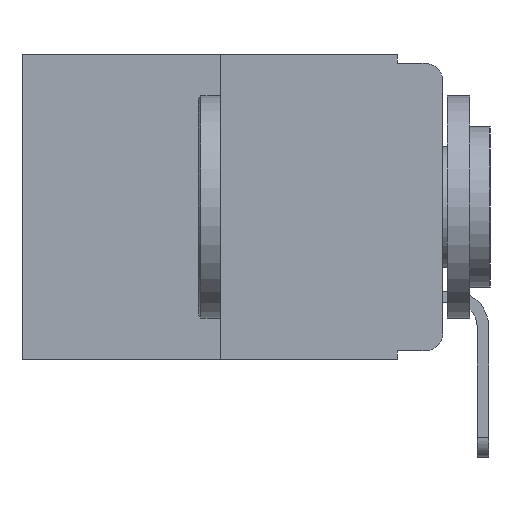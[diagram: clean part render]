
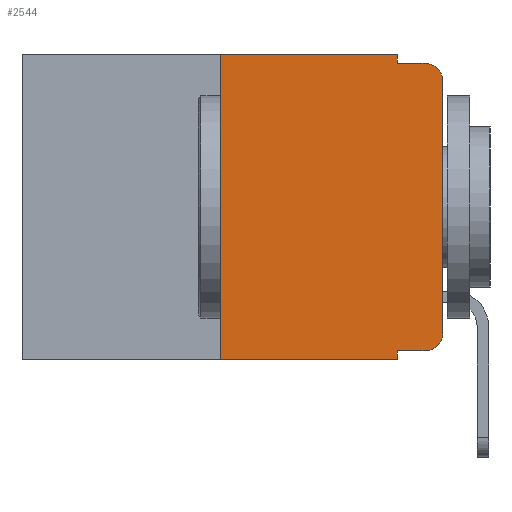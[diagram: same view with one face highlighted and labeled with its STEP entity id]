
A CAD part, left-side view. The second image highlights one B-rep face of the part: STEP entity #2544.
In plain terms, the highlighted planar face has unit normal (-1, 0, 0).
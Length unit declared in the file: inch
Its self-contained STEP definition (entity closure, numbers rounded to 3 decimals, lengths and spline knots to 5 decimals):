
#89 = VECTOR ( 'NONE', #8722, 39.37008 ) ;
#378 = AXIS2_PLACEMENT_3D ( 'NONE', #6134, #6126, #6123 ) ;
#442 = LINE ( 'NONE', #8966, #89 ) ;
#578 = VERTEX_POINT ( 'NONE', #7515 ) ;
#879 = ORIENTED_EDGE ( 'NONE', *, *, #8832, .T. ) ;
#962 = VERTEX_POINT ( 'NONE', #5371 ) ;
#1253 = ORIENTED_EDGE ( 'NONE', *, *, #8897, .T. ) ;
#1318 = CIRCLE ( 'NONE', #2718, 0.02 ) ;
#1372 = CARTESIAN_POINT ( 'NONE',  ( 0., 0.051, -0.333 ) ) ;
#1581 = CARTESIAN_POINT ( 'NONE',  ( 0., 0.25, -0.343 ) ) ;
#1769 = ORIENTED_EDGE ( 'NONE', *, *, #9022, .F. ) ;
#2022 = CARTESIAN_POINT ( 'NONE',  ( 0., 0., -0.313 ) ) ;
#2197 = ORIENTED_EDGE ( 'NONE', *, *, #9040, .F. ) ;
#2234 = ORIENTED_EDGE ( 'NONE', *, *, #4194, .F. ) ;
#2363 = CARTESIAN_POINT ( 'NONE',  ( 0., 0.051, -0.01 ) ) ;
#2544 = ADVANCED_FACE ( 'NONE', ( #10579 ), #7203, .F. ) ;
#2718 = AXIS2_PLACEMENT_3D ( 'NONE', #5008, #4945, #4886 ) ;
#2721 = CARTESIAN_POINT ( 'NONE',  ( 0., 0.051, -0.343 ) ) ;
#2747 = ORIENTED_EDGE ( 'NONE', *, *, #9093, .F. ) ;
#3010 = DIRECTION ( 'NONE',  ( 0., -1., 0. ) ) ;
#3046 = ORIENTED_EDGE ( 'NONE', *, *, #6772, .T. ) ;
#3079 = ORIENTED_EDGE ( 'NONE', *, *, #9110, .F. ) ;
#3125 = VERTEX_POINT ( 'NONE', #6711 ) ;
#3234 = EDGE_LOOP ( 'NONE', ( #879, #1253, #1769, #2197, #2234, #2747, #3046, #3079, #3517, #4168 ) ) ;
#3283 = LINE ( 'NONE', #8925, #7802 ) ;
#3517 = ORIENTED_EDGE ( 'NONE', *, *, #9247, .T. ) ;
#3841 = VECTOR ( 'NONE', #10121, 39.37008 ) ;
#3994 = CARTESIAN_POINT ( 'NONE',  ( 0., 0.051, 0. ) ) ;
#4105 = LINE ( 'NONE', #10224, #3841 ) ;
#4168 = ORIENTED_EDGE ( 'NONE', *, *, #9265, .T. ) ;
#4194 = EDGE_CURVE ( 'NONE', #962, #8372, #4105, .T. ) ;
#4379 = VECTOR ( 'NONE', #10527, 39.37008 ) ;
#4463 = CARTESIAN_POINT ( 'NONE',  ( 0., 0.473, -0.343 ) ) ;
#4886 = DIRECTION ( 'NONE',  ( 0., 0., -1. ) ) ;
#4945 = DIRECTION ( 'NONE',  ( -1., 0., 0. ) ) ;
#4958 = CARTESIAN_POINT ( 'NONE',  ( 0., 0.051, -0.01 ) ) ;
#5008 = CARTESIAN_POINT ( 'NONE',  ( 0., 0.02, -0.03 ) ) ;
#5371 = CARTESIAN_POINT ( 'NONE',  ( 0., 0.25, 0. ) ) ;
#5486 = CIRCLE ( 'NONE', #378, 0.02 ) ;
#5573 = VERTEX_POINT ( 'NONE', #2363 ) ;
#6052 = CARTESIAN_POINT ( 'NONE',  ( 0., 0.473, 0. ) ) ;
#6123 = DIRECTION ( 'NONE',  ( 0., 0., -1. ) ) ;
#6126 = DIRECTION ( 'NONE',  ( -1., 0., 0. ) ) ;
#6134 = CARTESIAN_POINT ( 'NONE',  ( 0., 0.02, -0.313 ) ) ;
#6207 = CARTESIAN_POINT ( 'NONE',  ( 0., 0., -0.03 ) ) ;
#6243 = DIRECTION ( 'NONE',  ( 0., -1., 0. ) ) ;
#6459 = CARTESIAN_POINT ( 'NONE',  ( 0., 0.051, -0.333 ) ) ;
#6471 = VERTEX_POINT ( 'NONE', #1581 ) ;
#6677 = LINE ( 'NONE', #11213, #4379 ) ;
#6703 = CARTESIAN_POINT ( 'NONE',  ( 0., 0., 0. ) ) ;
#6711 = CARTESIAN_POINT ( 'NONE',  ( 0., 0.02, -0.333 ) ) ;
#6740 = DIRECTION ( 'NONE',  ( 0., 0., 1. ) ) ;
#6772 = EDGE_CURVE ( 'NONE', #6471, #6805, #11391, .T. ) ;
#6805 = VERTEX_POINT ( 'NONE', #2721 ) ;
#6892 = VECTOR ( 'NONE', #11499, 39.37008 ) ;
#7203 = PLANE ( 'NONE',  #9797 ) ;
#7495 = DIRECTION ( 'NONE',  ( 1., 0., 0. ) ) ;
#7515 = CARTESIAN_POINT ( 'NONE',  ( 0., 0.02, -0.01 ) ) ;
#7655 = VECTOR ( 'NONE', #6243, 39.37008 ) ;
#7802 = VECTOR ( 'NONE', #8904, 39.37008 ) ;
#8372 = VERTEX_POINT ( 'NONE', #3994 ) ;
#8722 = DIRECTION ( 'NONE',  ( 0., 0., -1. ) ) ;
#8832 = EDGE_CURVE ( 'NONE', #10398, #9393, #11083, .T. ) ;
#8897 = EDGE_CURVE ( 'NONE', #9393, #578, #1318, .T. ) ;
#8904 = DIRECTION ( 'NONE',  ( 0., 0., 1. ) ) ;
#8925 = CARTESIAN_POINT ( 'NONE',  ( 0., 0.25, 0. ) ) ;
#8966 = CARTESIAN_POINT ( 'NONE',  ( 0., 0.051, 0. ) ) ;
#9022 = EDGE_CURVE ( 'NONE', #5573, #578, #9095, .T. ) ;
#9040 = EDGE_CURVE ( 'NONE', #8372, #5573, #6677, .T. ) ;
#9093 = EDGE_CURVE ( 'NONE', #6471, #962, #3283, .T. ) ;
#9095 = LINE ( 'NONE', #4958, #6892 ) ;
#9110 = EDGE_CURVE ( 'NONE', #11433, #6805, #442, .T. ) ;
#9240 = VECTOR ( 'NONE', #6740, 39.37008 ) ;
#9247 = EDGE_CURVE ( 'NONE', #11433, #3125, #9814, .T. ) ;
#9265 = EDGE_CURVE ( 'NONE', #3125, #10398, #5486, .T. ) ;
#9393 = VERTEX_POINT ( 'NONE', #6207 ) ;
#9500 = DIRECTION ( 'NONE',  ( 0., 0., -1. ) ) ;
#9797 = AXIS2_PLACEMENT_3D ( 'NONE', #6052, #7495, #9500 ) ;
#9814 = LINE ( 'NONE', #6459, #7655 ) ;
#10121 = DIRECTION ( 'NONE',  ( 0., -1., 0. ) ) ;
#10224 = CARTESIAN_POINT ( 'NONE',  ( 0., 0.473, 0. ) ) ;
#10398 = VERTEX_POINT ( 'NONE', #2022 ) ;
#10527 = DIRECTION ( 'NONE',  ( 0., 0., -1. ) ) ;
#10579 = FACE_OUTER_BOUND ( 'NONE', #3234, .T. ) ;
#11083 = LINE ( 'NONE', #6703, #9240 ) ;
#11118 = VECTOR ( 'NONE', #3010, 39.37008 ) ;
#11213 = CARTESIAN_POINT ( 'NONE',  ( 0., 0.051, 0. ) ) ;
#11391 = LINE ( 'NONE', #4463, #11118 ) ;
#11433 = VERTEX_POINT ( 'NONE', #1372 ) ;
#11499 = DIRECTION ( 'NONE',  ( 0., -1., 0. ) ) ;
